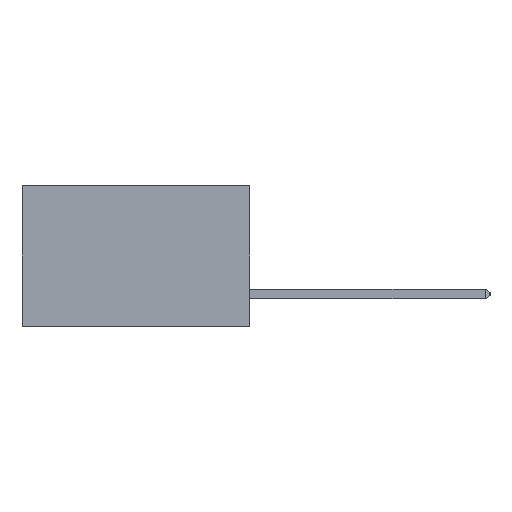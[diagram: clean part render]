
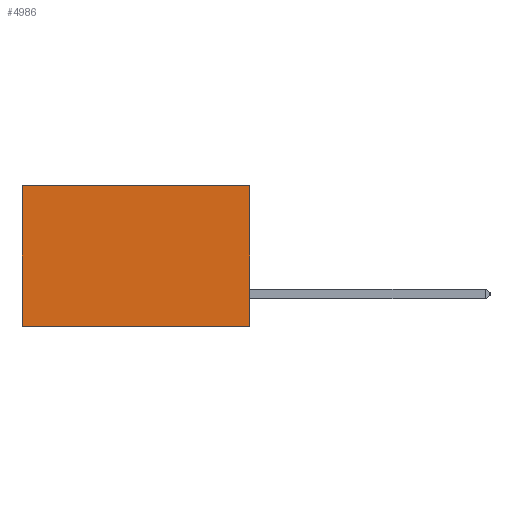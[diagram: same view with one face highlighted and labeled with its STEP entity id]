
A CAD part, left-side view. The second image highlights one B-rep face of the part: STEP entity #4986.
In plain terms, the highlighted planar face has unit normal (-1, 0, 0).
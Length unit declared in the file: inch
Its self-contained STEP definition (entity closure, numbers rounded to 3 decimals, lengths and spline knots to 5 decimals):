
#216 = EDGE_CURVE ( 'NONE', #8873, #1479, #7438, .T. ) ;
#307 = ORIENTED_EDGE ( 'NONE', *, *, #216, .F. ) ;
#358 = LINE ( 'NONE', #5158, #4973 ) ;
#1275 = DIRECTION ( 'NONE',  ( 0., 0., -1. ) ) ;
#1479 = VERTEX_POINT ( 'NONE', #6865 ) ;
#1793 = CARTESIAN_POINT ( 'NONE',  ( 0.2875, 0., 0. ) ) ;
#2326 = VECTOR ( 'NONE', #1275, 39.37008 ) ;
#2748 = CARTESIAN_POINT ( 'NONE',  ( 0.2875, 0., -0.37 ) ) ;
#3150 = EDGE_CURVE ( 'NONE', #4122, #8873, #11678, .T. ) ;
#3194 = DIRECTION ( 'NONE',  ( 0., 0., -1. ) ) ;
#3752 = ORIENTED_EDGE ( 'NONE', *, *, #4941, .T. ) ;
#4122 = VERTEX_POINT ( 'NONE', #1793 ) ;
#4666 = DIRECTION ( 'NONE',  ( 0., 0., -1. ) ) ;
#4675 = DIRECTION ( 'NONE',  ( 1., 0., 0. ) ) ;
#4689 = CARTESIAN_POINT ( 'NONE',  ( 0.2875, 0., 0. ) ) ;
#4761 = PLANE ( 'NONE',  #10160 ) ;
#4936 = VECTOR ( 'NONE', #6958, 39.37008 ) ;
#4941 = EDGE_CURVE ( 'NONE', #4122, #10120, #358, .T. ) ;
#4973 = VECTOR ( 'NONE', #5171, 39.37008 ) ;
#4986 = ADVANCED_FACE ( 'NONE', ( #6886 ), #4761, .F. ) ;
#5017 = CARTESIAN_POINT ( 'NONE',  ( 0.2875, 0., 0. ) ) ;
#5158 = CARTESIAN_POINT ( 'NONE',  ( 0.2875, 0., 0. ) ) ;
#5171 = DIRECTION ( 'NONE',  ( 0., 1., 0. ) ) ;
#6022 = CARTESIAN_POINT ( 'NONE',  ( 0.2875, 0.6, 0. ) ) ;
#6138 = CARTESIAN_POINT ( 'NONE',  ( 0.2875, 0.6, 0. ) ) ;
#6282 = ORIENTED_EDGE ( 'NONE', *, *, #3150, .F. ) ;
#6865 = CARTESIAN_POINT ( 'NONE',  ( 0.2875, 0.6, -0.37 ) ) ;
#6886 = FACE_OUTER_BOUND ( 'NONE', #11652, .T. ) ;
#6958 = DIRECTION ( 'NONE',  ( 0., 1., 0. ) ) ;
#7438 = LINE ( 'NONE', #9230, #4936 ) ;
#8582 = EDGE_CURVE ( 'NONE', #10120, #1479, #9672, .T. ) ;
#8873 = VERTEX_POINT ( 'NONE', #2748 ) ;
#9230 = CARTESIAN_POINT ( 'NONE',  ( 0.2875, 0., -0.37 ) ) ;
#9603 = VECTOR ( 'NONE', #3194, 39.37008 ) ;
#9672 = LINE ( 'NONE', #6138, #2326 ) ;
#10120 = VERTEX_POINT ( 'NONE', #6022 ) ;
#10160 = AXIS2_PLACEMENT_3D ( 'NONE', #4689, #4675, #4666 ) ;
#10926 = ORIENTED_EDGE ( 'NONE', *, *, #8582, .T. ) ;
#11652 = EDGE_LOOP ( 'NONE', ( #10926, #307, #6282, #3752 ) ) ;
#11678 = LINE ( 'NONE', #5017, #9603 ) ;
